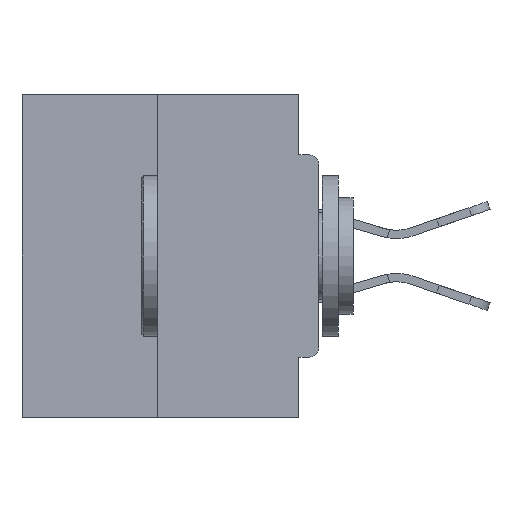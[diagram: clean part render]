
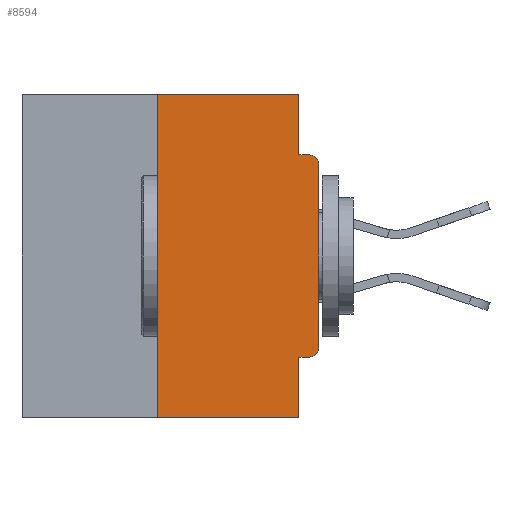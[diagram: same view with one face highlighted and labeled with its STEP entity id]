
A CAD part, left-side view. The second image highlights one B-rep face of the part: STEP entity #8594.
In plain terms, the highlighted planar face has unit normal (-1, 0, 0).
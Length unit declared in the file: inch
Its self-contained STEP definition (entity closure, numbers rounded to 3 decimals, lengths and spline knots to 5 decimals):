
#213 = VERTEX_POINT ( 'NONE', #27045 ) ;
#532 = VECTOR ( 'NONE', #31513, 39.37008 ) ;
#902 = CARTESIAN_POINT ( 'NONE',  ( 0., 0.031, -0.4065 ) ) ;
#1869 = VERTEX_POINT ( 'NONE', #10547 ) ;
#2083 = CARTESIAN_POINT ( 'NONE',  ( 0., 0.015, -0.3915 ) ) ;
#2393 = CARTESIAN_POINT ( 'NONE',  ( 0., 0., 0. ) ) ;
#2448 = LINE ( 'NONE', #6780, #532 ) ;
#2611 = ORIENTED_EDGE ( 'NONE', *, *, #22323, .F. ) ;
#2864 = VERTEX_POINT ( 'NONE', #32608 ) ;
#3449 = VECTOR ( 'NONE', #16806, 39.37008 ) ;
#3965 = ORIENTED_EDGE ( 'NONE', *, *, #27718, .T. ) ;
#4052 = VECTOR ( 'NONE', #16444, 39.37008 ) ;
#4549 = CARTESIAN_POINT ( 'NONE',  ( 0., 0.031, -0.5 ) ) ;
#4653 = ORIENTED_EDGE ( 'NONE', *, *, #14410, .T. ) ;
#5293 = DIRECTION ( 'NONE',  ( 0., 0., -1. ) ) ;
#5842 = EDGE_CURVE ( 'NONE', #18259, #20754, #32516, .T. ) ;
#6236 = ORIENTED_EDGE ( 'NONE', *, *, #13071, .F. ) ;
#6540 = AXIS2_PLACEMENT_3D ( 'NONE', #19327, #18800, #6955 ) ;
#6780 = CARTESIAN_POINT ( 'NONE',  ( 0., 0.46, -0.5 ) ) ;
#6955 = DIRECTION ( 'NONE',  ( 0., 0., -1. ) ) ;
#6983 = VERTEX_POINT ( 'NONE', #35348 ) ;
#7018 = AXIS2_PLACEMENT_3D ( 'NONE', #22326, #25226, #21950 ) ;
#7899 = ORIENTED_EDGE ( 'NONE', *, *, #9912, .T. ) ;
#8594 = ADVANCED_FACE ( 'NONE', ( #29902 ), #12897, .F. ) ;
#9912 = EDGE_CURVE ( 'NONE', #18690, #20754, #2448, .T. ) ;
#10547 = CARTESIAN_POINT ( 'NONE',  ( 0., 0.25, 0. ) ) ;
#10575 = LINE ( 'NONE', #28552, #21060 ) ;
#12897 = PLANE ( 'NONE',  #7018 ) ;
#13071 = EDGE_CURVE ( 'NONE', #37594, #6983, #18820, .T. ) ;
#13204 = VERTEX_POINT ( 'NONE', #14042 ) ;
#13267 = AXIS2_PLACEMENT_3D ( 'NONE', #2083, #17401, #5293 ) ;
#14042 = CARTESIAN_POINT ( 'NONE',  ( 0., 0.031, 0. ) ) ;
#14198 = ORIENTED_EDGE ( 'NONE', *, *, #23873, .F. ) ;
#14410 = EDGE_CURVE ( 'NONE', #2864, #29156, #16340, .T. ) ;
#15488 = CARTESIAN_POINT ( 'NONE',  ( 0., 0.031, -0.5 ) ) ;
#16271 = CARTESIAN_POINT ( 'NONE',  ( 0., 0.031, -0.0935 ) ) ;
#16340 = LINE ( 'NONE', #2393, #34884 ) ;
#16444 = DIRECTION ( 'NONE',  ( 0., -1., 0. ) ) ;
#16806 = DIRECTION ( 'NONE',  ( 0., 0., -1. ) ) ;
#16916 = CARTESIAN_POINT ( 'NONE',  ( 0., 0., -0.4065 ) ) ;
#17401 = DIRECTION ( 'NONE',  ( -1., 0., 0. ) ) ;
#18259 = VERTEX_POINT ( 'NONE', #902 ) ;
#18690 = VERTEX_POINT ( 'NONE', #24443 ) ;
#18800 = DIRECTION ( 'NONE',  ( -1., 0., 0. ) ) ;
#18820 = LINE ( 'NONE', #22812, #4052 ) ;
#19327 = CARTESIAN_POINT ( 'NONE',  ( 0., 0.015, -0.1085 ) ) ;
#19996 = DIRECTION ( 'NONE',  ( 0., 1., 0. ) ) ;
#20109 = EDGE_CURVE ( 'NONE', #29156, #6983, #34950, .T. ) ;
#20754 = VERTEX_POINT ( 'NONE', #15488 ) ;
#21060 = VECTOR ( 'NONE', #25636, 39.37008 ) ;
#21334 = DIRECTION ( 'NONE',  ( 0., 0., -1. ) ) ;
#21918 = LINE ( 'NONE', #22494, #29022 ) ;
#21944 = LINE ( 'NONE', #32632, #29049 ) ;
#21950 = DIRECTION ( 'NONE',  ( 0., 0., -1. ) ) ;
#22323 = EDGE_CURVE ( 'NONE', #1869, #13204, #21918, .T. ) ;
#22326 = CARTESIAN_POINT ( 'NONE',  ( 0., 0.46, 0. ) ) ;
#22494 = CARTESIAN_POINT ( 'NONE',  ( 0., 0.46, 0. ) ) ;
#22812 = CARTESIAN_POINT ( 'NONE',  ( 0., 0., -0.0935 ) ) ;
#23658 = LINE ( 'NONE', #16916, #34126 ) ;
#23873 = EDGE_CURVE ( 'NONE', #18690, #1869, #10575, .T. ) ;
#24443 = CARTESIAN_POINT ( 'NONE',  ( 0., 0.25, -0.5 ) ) ;
#25226 = DIRECTION ( 'NONE',  ( 1., 0., 0. ) ) ;
#25534 = CIRCLE ( 'NONE', #13267, 0.015 ) ;
#25636 = DIRECTION ( 'NONE',  ( 0., 0., 1. ) ) ;
#25748 = EDGE_CURVE ( 'NONE', #13204, #37594, #21944, .T. ) ;
#26992 = ORIENTED_EDGE ( 'NONE', *, *, #25748, .F. ) ;
#27045 = CARTESIAN_POINT ( 'NONE',  ( 0., 0.015, -0.4065 ) ) ;
#27718 = EDGE_CURVE ( 'NONE', #213, #2864, #25534, .T. ) ;
#28552 = CARTESIAN_POINT ( 'NONE',  ( 0., 0.25, 0. ) ) ;
#28697 = ORIENTED_EDGE ( 'NONE', *, *, #5842, .F. ) ;
#29022 = VECTOR ( 'NONE', #31940, 39.37008 ) ;
#29049 = VECTOR ( 'NONE', #21334, 39.37008 ) ;
#29156 = VERTEX_POINT ( 'NONE', #35183 ) ;
#29902 = FACE_OUTER_BOUND ( 'NONE', #31782, .T. ) ;
#31513 = DIRECTION ( 'NONE',  ( 0., -1., 0. ) ) ;
#31782 = EDGE_LOOP ( 'NONE', ( #2611, #14198, #7899, #28697, #32001, #3965, #4653, #34400, #6236, #26992 ) ) ;
#31940 = DIRECTION ( 'NONE',  ( 0., -1., 0. ) ) ;
#32001 = ORIENTED_EDGE ( 'NONE', *, *, #34695, .F. ) ;
#32516 = LINE ( 'NONE', #4549, #3449 ) ;
#32608 = CARTESIAN_POINT ( 'NONE',  ( 0., 0., -0.3915 ) ) ;
#32632 = CARTESIAN_POINT ( 'NONE',  ( 0., 0.031, 0. ) ) ;
#34126 = VECTOR ( 'NONE', #19996, 39.37008 ) ;
#34400 = ORIENTED_EDGE ( 'NONE', *, *, #20109, .T. ) ;
#34695 = EDGE_CURVE ( 'NONE', #213, #18259, #23658, .T. ) ;
#34884 = VECTOR ( 'NONE', #38632, 39.37008 ) ;
#34950 = CIRCLE ( 'NONE', #6540, 0.015 ) ;
#35183 = CARTESIAN_POINT ( 'NONE',  ( 0., 0., -0.1085 ) ) ;
#35348 = CARTESIAN_POINT ( 'NONE',  ( 0., 0.015, -0.0935 ) ) ;
#37594 = VERTEX_POINT ( 'NONE', #16271 ) ;
#38632 = DIRECTION ( 'NONE',  ( 0., 0., 1. ) ) ;
